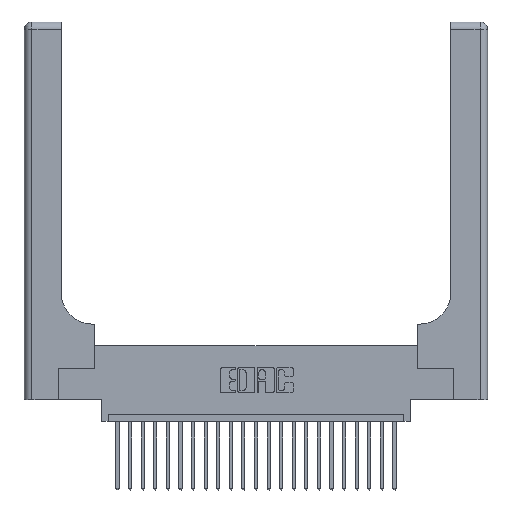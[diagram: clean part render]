
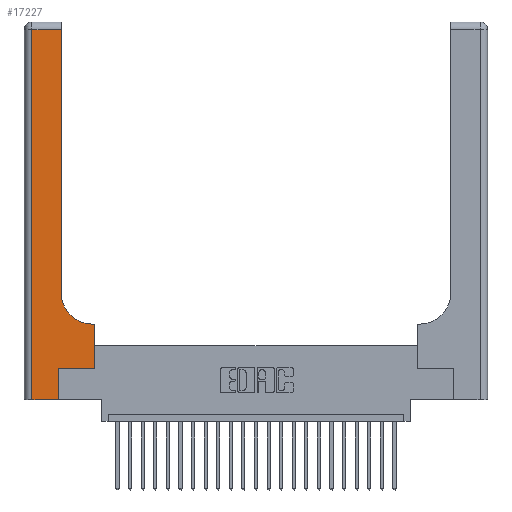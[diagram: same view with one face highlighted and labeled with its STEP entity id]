
A CAD part, top view. The second image highlights one B-rep face of the part: STEP entity #17227.
In plain terms, the highlighted planar face has unit normal (0, 0, 1).
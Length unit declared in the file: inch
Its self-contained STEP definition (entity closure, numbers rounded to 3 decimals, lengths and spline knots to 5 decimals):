
#378 = DIRECTION ( 'NONE',  ( 1., 0., 0. ) ) ;
#629 = VECTOR ( 'NONE', #16187, 39.37008 ) ;
#806 = VECTOR ( 'NONE', #378, 39.37008 ) ;
#1686 = CARTESIAN_POINT ( 'NONE',  ( 0., 2.94, 0.37 ) ) ;
#2110 = VERTEX_POINT ( 'NONE', #24638 ) ;
#2232 = CARTESIAN_POINT ( 'NONE',  ( 0.5415, 0.6, 0.37 ) ) ;
#2636 = AXIS2_PLACEMENT_3D ( 'NONE', #13231, #3452, #3539 ) ;
#2692 = VERTEX_POINT ( 'NONE', #10471 ) ;
#2763 = ORIENTED_EDGE ( 'NONE', *, *, #15193, .T. ) ;
#2892 = AXIS2_PLACEMENT_3D ( 'NONE', #14734, #6828, #10799 ) ;
#2937 = ORIENTED_EDGE ( 'NONE', *, *, #14769, .T. ) ;
#3059 = CARTESIAN_POINT ( 'NONE',  ( 0.2915, 0.6, 0.37 ) ) ;
#3374 = PLANE ( 'NONE',  #2636 ) ;
#3452 = DIRECTION ( 'NONE',  ( 0., 0., -1. ) ) ;
#3539 = DIRECTION ( 'NONE',  ( -1., 0., 0. ) ) ;
#4344 = VERTEX_POINT ( 'NONE', #19602 ) ;
#6560 = DIRECTION ( 'NONE',  ( 0., -1., 0. ) ) ;
#6763 = ORIENTED_EDGE ( 'NONE', *, *, #18226, .T. ) ;
#6828 = DIRECTION ( 'NONE',  ( 0., 0., -1. ) ) ;
#7087 = VERTEX_POINT ( 'NONE', #18004 ) ;
#7332 = LINE ( 'NONE', #12511, #20763 ) ;
#7475 = DIRECTION ( 'NONE',  ( -1., 0., 0. ) ) ;
#8006 = CARTESIAN_POINT ( 'NONE',  ( 0.269, 0.25, 0.37 ) ) ;
#8477 = CARTESIAN_POINT ( 'NONE',  ( 0.5585, 0.25, 0.37 ) ) ;
#8512 = VECTOR ( 'NONE', #22949, 39.37008 ) ;
#8719 = LINE ( 'NONE', #8006, #806 ) ;
#8938 = DIRECTION ( 'NONE',  ( -1., 0., 0. ) ) ;
#9061 = FACE_OUTER_BOUND ( 'NONE', #16250, .T. ) ;
#9395 = ORIENTED_EDGE ( 'NONE', *, *, #9458, .T. ) ;
#9458 = EDGE_CURVE ( 'NONE', #4344, #15197, #23492, .T. ) ;
#9711 = EDGE_CURVE ( 'NONE', #2110, #13077, #12765, .T. ) ;
#10471 = CARTESIAN_POINT ( 'NONE',  ( 0.269, 0.25, 0.37 ) ) ;
#10608 = VERTEX_POINT ( 'NONE', #2232 ) ;
#10668 = VECTOR ( 'NONE', #7475, 39.37008 ) ;
#10799 = DIRECTION ( 'NONE',  ( 1., 0., 0. ) ) ;
#11274 = EDGE_CURVE ( 'NONE', #2692, #4344, #8719, .T. ) ;
#12232 = ORIENTED_EDGE ( 'NONE', *, *, #24980, .T. ) ;
#12511 = CARTESIAN_POINT ( 'NONE',  ( 0.06, 3., 0.37 ) ) ;
#12765 = LINE ( 'NONE', #12805, #8512 ) ;
#12805 = CARTESIAN_POINT ( 'NONE',  ( 0.2915, 3., 0.37 ) ) ;
#13077 = VERTEX_POINT ( 'NONE', #20675 ) ;
#13231 = CARTESIAN_POINT ( 'NONE',  ( 0., 3., 0.37 ) ) ;
#13802 = CARTESIAN_POINT ( 'NONE',  ( 0.06, 2.94, 0.37 ) ) ;
#14734 = CARTESIAN_POINT ( 'NONE',  ( 0.5415, 0.85, 0.37 ) ) ;
#14769 = EDGE_CURVE ( 'NONE', #20111, #17893, #7332, .T. ) ;
#14934 = LINE ( 'NONE', #1686, #10668 ) ;
#15193 = EDGE_CURVE ( 'NONE', #13077, #20111, #14934, .T. ) ;
#15197 = VERTEX_POINT ( 'NONE', #17704 ) ;
#15309 = CARTESIAN_POINT ( 'NONE',  ( 0.06, 0., 0.37 ) ) ;
#16187 = DIRECTION ( 'NONE',  ( 1., 0., 0. ) ) ;
#16209 = EDGE_CURVE ( 'NONE', #10608, #2110, #21297, .T. ) ;
#16250 = EDGE_LOOP ( 'NONE', ( #19095, #2763, #2937, #19746, #12232, #21042, #9395, #6763, #24407 ) ) ;
#16310 = VECTOR ( 'NONE', #8938, 39.37008 ) ;
#17227 = ADVANCED_FACE ( 'NONE', ( #9061 ), #3374, .F. ) ;
#17344 = LINE ( 'NONE', #23016, #24375 ) ;
#17704 = CARTESIAN_POINT ( 'NONE',  ( 0.5585, 0.6, 0.37 ) ) ;
#17893 = VERTEX_POINT ( 'NONE', #15309 ) ;
#18004 = CARTESIAN_POINT ( 'NONE',  ( 0.269, 0., 0.37 ) ) ;
#18069 = CARTESIAN_POINT ( 'NONE',  ( 0., 0., 0.37 ) ) ;
#18226 = EDGE_CURVE ( 'NONE', #15197, #10608, #24563, .T. ) ;
#18609 = VECTOR ( 'NONE', #23724, 39.37008 ) ;
#19095 = ORIENTED_EDGE ( 'NONE', *, *, #9711, .T. ) ;
#19602 = CARTESIAN_POINT ( 'NONE',  ( 0.5585, 0.25, 0.37 ) ) ;
#19746 = ORIENTED_EDGE ( 'NONE', *, *, #22008, .T. ) ;
#20111 = VERTEX_POINT ( 'NONE', #13802 ) ;
#20675 = CARTESIAN_POINT ( 'NONE',  ( 0.2915, 2.94, 0.37 ) ) ;
#20763 = VECTOR ( 'NONE', #6560, 39.37008 ) ;
#20878 = DIRECTION ( 'NONE',  ( 0., 1., 0. ) ) ;
#21042 = ORIENTED_EDGE ( 'NONE', *, *, #11274, .T. ) ;
#21297 = CIRCLE ( 'NONE', #2892, 0.25 ) ;
#21337 = LINE ( 'NONE', #18069, #629 ) ;
#22008 = EDGE_CURVE ( 'NONE', #17893, #7087, #21337, .T. ) ;
#22949 = DIRECTION ( 'NONE',  ( 0., 1., 0. ) ) ;
#23016 = CARTESIAN_POINT ( 'NONE',  ( 0.269, 0., 0.37 ) ) ;
#23492 = LINE ( 'NONE', #8477, #18609 ) ;
#23724 = DIRECTION ( 'NONE',  ( 0., 1., 0. ) ) ;
#24375 = VECTOR ( 'NONE', #20878, 39.37008 ) ;
#24407 = ORIENTED_EDGE ( 'NONE', *, *, #16209, .T. ) ;
#24563 = LINE ( 'NONE', #3059, #16310 ) ;
#24638 = CARTESIAN_POINT ( 'NONE',  ( 0.2915, 0.85, 0.37 ) ) ;
#24980 = EDGE_CURVE ( 'NONE', #7087, #2692, #17344, .T. ) ;
